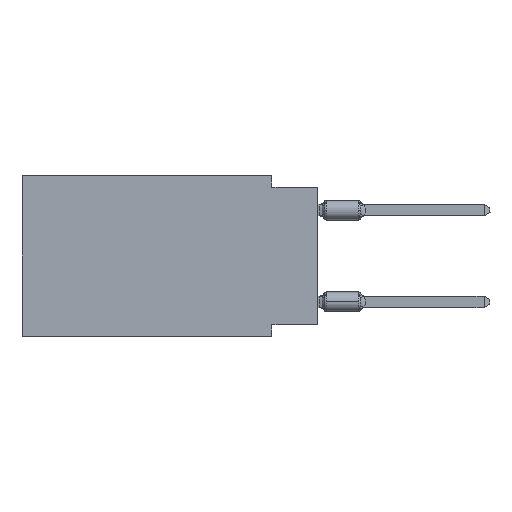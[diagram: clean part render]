
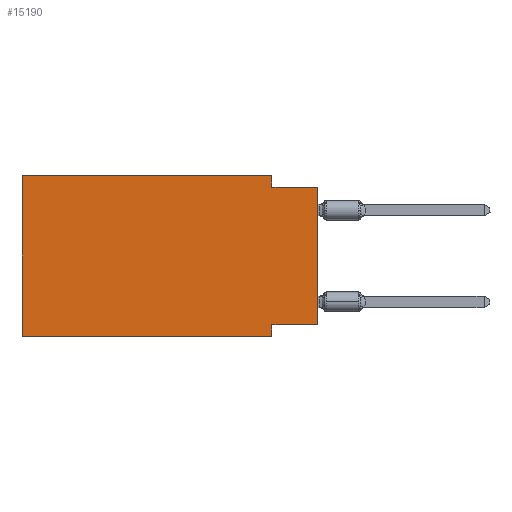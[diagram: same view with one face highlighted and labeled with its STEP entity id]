
A CAD part, left-side view. The second image highlights one B-rep face of the part: STEP entity #15190.
In plain terms, the highlighted planar face has unit normal (-1, 0, 0).
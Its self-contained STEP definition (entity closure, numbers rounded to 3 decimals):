
#122 = VERTEX_POINT ( 'NONE', #7014 ) ;
#174 = EDGE_CURVE ( 'NONE', #32867, #21375, #28732, .T. ) ;
#313 = AXIS2_PLACEMENT_3D ( 'NONE', #30935, #33966, #3382 ) ;
#873 = EDGE_CURVE ( 'NONE', #122, #28932, #9145, .T. ) ;
#2361 = CARTESIAN_POINT ( 'NONE',  ( 0., 16.383, -8.89 ) ) ;
#2559 = VECTOR ( 'NONE', #37779, 1000. ) ;
#2664 = VECTOR ( 'NONE', #37322, 1000. ) ;
#3382 = DIRECTION ( 'NONE',  ( 0., 0., -1. ) ) ;
#3418 = ORIENTED_EDGE ( 'NONE', *, *, #34983, .T. ) ;
#3742 = CARTESIAN_POINT ( 'NONE',  ( 0., 16.383, 0. ) ) ;
#3775 = LINE ( 'NONE', #25490, #38914 ) ;
#4397 = CARTESIAN_POINT ( 'NONE',  ( 0., 16.383, 0. ) ) ;
#5729 = CARTESIAN_POINT ( 'NONE',  ( 0., 2.54, 0. ) ) ;
#6411 = FACE_OUTER_BOUND ( 'NONE', #11622, .T. ) ;
#6864 = VERTEX_POINT ( 'NONE', #25470 ) ;
#7014 = CARTESIAN_POINT ( 'NONE',  ( 0., 2.54, -0.635 ) ) ;
#7340 = DIRECTION ( 'NONE',  ( 0., 0., -1. ) ) ;
#8391 = VECTOR ( 'NONE', #14994, 1000. ) ;
#9145 = LINE ( 'NONE', #14804, #8391 ) ;
#9973 = LINE ( 'NONE', #22036, #38170 ) ;
#9980 = LINE ( 'NONE', #3742, #2664 ) ;
#10441 = DIRECTION ( 'NONE',  ( 0., 0., -1. ) ) ;
#11151 = VERTEX_POINT ( 'NONE', #23254 ) ;
#11622 = EDGE_LOOP ( 'NONE', ( #29971, #11910, #18422, #36806, #34517, #3418, #23396, #39500 ) ) ;
#11910 = ORIENTED_EDGE ( 'NONE', *, *, #873, .F. ) ;
#14777 = DIRECTION ( 'NONE',  ( 0., 0., 1. ) ) ;
#14804 = CARTESIAN_POINT ( 'NONE',  ( 0., 0., -0.635 ) ) ;
#14994 = DIRECTION ( 'NONE',  ( 0., -1., 0. ) ) ;
#15190 = ADVANCED_FACE ( 'NONE', ( #6411 ), #22089, .F. ) ;
#15547 = VECTOR ( 'NONE', #17953, 1000. ) ;
#16238 = DIRECTION ( 'NONE',  ( 0., -1., 0. ) ) ;
#16882 = LINE ( 'NONE', #34972, #35583 ) ;
#16925 = EDGE_CURVE ( 'NONE', #21375, #17276, #9980, .T. ) ;
#17276 = VERTEX_POINT ( 'NONE', #5729 ) ;
#17588 = CARTESIAN_POINT ( 'NONE',  ( 0., 0., 0. ) ) ;
#17953 = DIRECTION ( 'NONE',  ( 0., 1., 0. ) ) ;
#18422 = ORIENTED_EDGE ( 'NONE', *, *, #31038, .F. ) ;
#21375 = VERTEX_POINT ( 'NONE', #28331 ) ;
#22036 = CARTESIAN_POINT ( 'NONE',  ( 0., 2.54, -8.89 ) ) ;
#22089 = PLANE ( 'NONE',  #313 ) ;
#23254 = CARTESIAN_POINT ( 'NONE',  ( 0., 2.54, -8.89 ) ) ;
#23396 = ORIENTED_EDGE ( 'NONE', *, *, #29826, .F. ) ;
#23578 = CARTESIAN_POINT ( 'NONE',  ( 0., 2.54, -8.255 ) ) ;
#23761 = VERTEX_POINT ( 'NONE', #23578 ) ;
#24190 = LINE ( 'NONE', #30023, #15547 ) ;
#25470 = CARTESIAN_POINT ( 'NONE',  ( 0., 0., -8.255 ) ) ;
#25490 = CARTESIAN_POINT ( 'NONE',  ( 0., 16.383, -8.89 ) ) ;
#28331 = CARTESIAN_POINT ( 'NONE',  ( 0., 16.383, 0. ) ) ;
#28732 = LINE ( 'NONE', #4397, #2559 ) ;
#28932 = VERTEX_POINT ( 'NONE', #32168 ) ;
#29826 = EDGE_CURVE ( 'NONE', #23761, #11151, #9973, .T. ) ;
#29971 = ORIENTED_EDGE ( 'NONE', *, *, #34336, .T. ) ;
#30023 = CARTESIAN_POINT ( 'NONE',  ( 0., 0., -8.255 ) ) ;
#30935 = CARTESIAN_POINT ( 'NONE',  ( 0., 16.383, 0. ) ) ;
#31038 = EDGE_CURVE ( 'NONE', #17276, #122, #16882, .T. ) ;
#32168 = CARTESIAN_POINT ( 'NONE',  ( 0., 0., -0.635 ) ) ;
#32867 = VERTEX_POINT ( 'NONE', #2361 ) ;
#32870 = LINE ( 'NONE', #17588, #38711 ) ;
#33344 = EDGE_CURVE ( 'NONE', #6864, #23761, #24190, .T. ) ;
#33966 = DIRECTION ( 'NONE',  ( 1., 0., 0. ) ) ;
#34336 = EDGE_CURVE ( 'NONE', #6864, #28932, #32870, .T. ) ;
#34517 = ORIENTED_EDGE ( 'NONE', *, *, #174, .F. ) ;
#34972 = CARTESIAN_POINT ( 'NONE',  ( 0., 2.54, 0. ) ) ;
#34983 = EDGE_CURVE ( 'NONE', #32867, #11151, #3775, .T. ) ;
#35583 = VECTOR ( 'NONE', #10441, 1000. ) ;
#36806 = ORIENTED_EDGE ( 'NONE', *, *, #16925, .F. ) ;
#37322 = DIRECTION ( 'NONE',  ( 0., -1., 0. ) ) ;
#37779 = DIRECTION ( 'NONE',  ( 0., 0., 1. ) ) ;
#38170 = VECTOR ( 'NONE', #7340, 1000. ) ;
#38711 = VECTOR ( 'NONE', #14777, 1000. ) ;
#38914 = VECTOR ( 'NONE', #16238, 1000. ) ;
#39500 = ORIENTED_EDGE ( 'NONE', *, *, #33344, .F. ) ;
